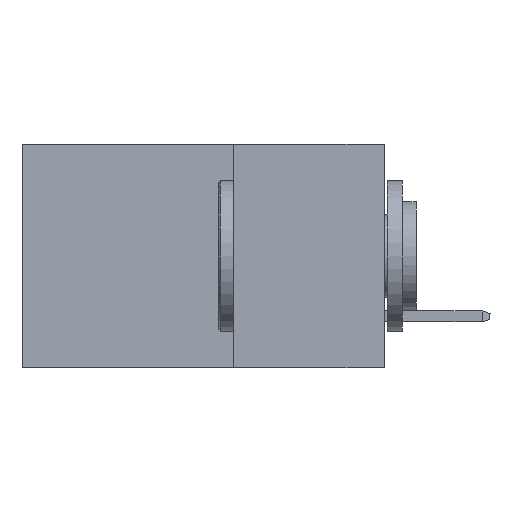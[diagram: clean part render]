
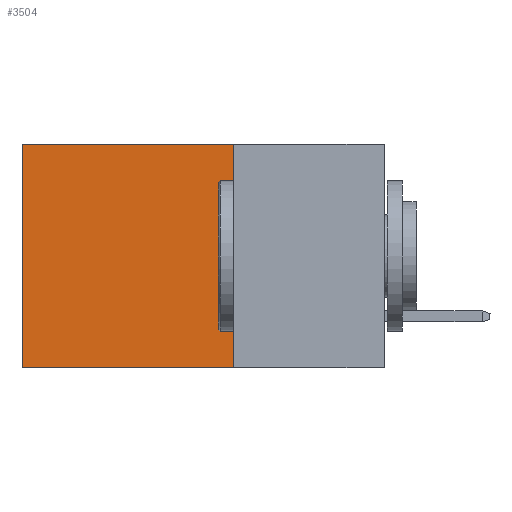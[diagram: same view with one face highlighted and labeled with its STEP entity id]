
A CAD part, left-side view. The second image highlights one B-rep face of the part: STEP entity #3504.
In plain terms, the highlighted planar face has unit normal (-1, 0, 0).
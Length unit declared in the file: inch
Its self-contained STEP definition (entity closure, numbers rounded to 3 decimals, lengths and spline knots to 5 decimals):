
#85 = LINE ( 'NONE', #8785, #5716 ) ;
#1311 = VERTEX_POINT ( 'NONE', #5782 ) ;
#2028 = CARTESIAN_POINT ( 'NONE',  ( 0.2615, 0.6, 0. ) ) ;
#2084 = DIRECTION ( 'NONE',  ( 0., 0., -1. ) ) ;
#2278 = ORIENTED_EDGE ( 'NONE', *, *, #8226, .F. ) ;
#2603 = FACE_OUTER_BOUND ( 'NONE', #5898, .T. ) ;
#3267 = VERTEX_POINT ( 'NONE', #8918 ) ;
#3408 = LINE ( 'NONE', #9093, #4354 ) ;
#3456 = DIRECTION ( 'NONE',  ( 0., 0., -1. ) ) ;
#3504 = ADVANCED_FACE ( 'NONE', ( #2603 ), #5844, .F. ) ;
#3590 = DIRECTION ( 'NONE',  ( 0., 1., 0. ) ) ;
#3896 = AXIS2_PLACEMENT_3D ( 'NONE', #9090, #10261, #2084 ) ;
#4238 = ORIENTED_EDGE ( 'NONE', *, *, #6737, .T. ) ;
#4354 = VECTOR ( 'NONE', #3456, 39.37008 ) ;
#4796 = DIRECTION ( 'NONE',  ( 0., 1., 0. ) ) ;
#5182 = LINE ( 'NONE', #8441, #5242 ) ;
#5242 = VECTOR ( 'NONE', #3590, 39.37008 ) ;
#5301 = LINE ( 'NONE', #5509, #8673 ) ;
#5509 = CARTESIAN_POINT ( 'NONE',  ( 0.2615, 0.25, -0.37 ) ) ;
#5526 = VERTEX_POINT ( 'NONE', #7730 ) ;
#5629 = ORIENTED_EDGE ( 'NONE', *, *, #9774, .T. ) ;
#5716 = VECTOR ( 'NONE', #4796, 39.37008 ) ;
#5782 = CARTESIAN_POINT ( 'NONE',  ( 0.2615, 0.25, -0.37 ) ) ;
#5844 = PLANE ( 'NONE',  #3896 ) ;
#5898 = EDGE_LOOP ( 'NONE', ( #5629, #10231, #2278, #4238 ) ) ;
#6318 = EDGE_CURVE ( 'NONE', #1311, #5526, #85, .T. ) ;
#6737 = EDGE_CURVE ( 'NONE', #3267, #9338, #5182, .T. ) ;
#7730 = CARTESIAN_POINT ( 'NONE',  ( 0.2615, 0.6, -0.37 ) ) ;
#7805 = DIRECTION ( 'NONE',  ( 0., 0., -1. ) ) ;
#8226 = EDGE_CURVE ( 'NONE', #3267, #1311, #5301, .T. ) ;
#8441 = CARTESIAN_POINT ( 'NONE',  ( 0.2615, 0.25, 0. ) ) ;
#8673 = VECTOR ( 'NONE', #7805, 39.37008 ) ;
#8785 = CARTESIAN_POINT ( 'NONE',  ( 0.2615, 0.25, -0.37 ) ) ;
#8918 = CARTESIAN_POINT ( 'NONE',  ( 0.2615, 0.25, 0. ) ) ;
#9090 = CARTESIAN_POINT ( 'NONE',  ( 0.2615, 0.25, -0.37 ) ) ;
#9093 = CARTESIAN_POINT ( 'NONE',  ( 0.2615, 0.6, -0.37 ) ) ;
#9338 = VERTEX_POINT ( 'NONE', #2028 ) ;
#9774 = EDGE_CURVE ( 'NONE', #9338, #5526, #3408, .T. ) ;
#10231 = ORIENTED_EDGE ( 'NONE', *, *, #6318, .F. ) ;
#10261 = DIRECTION ( 'NONE',  ( 1., 0., 0. ) ) ;
